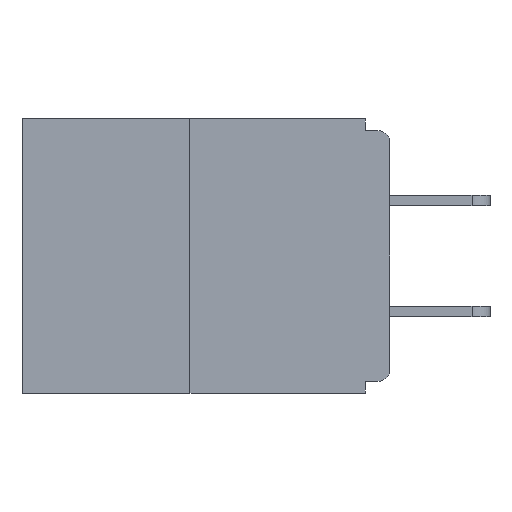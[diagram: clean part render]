
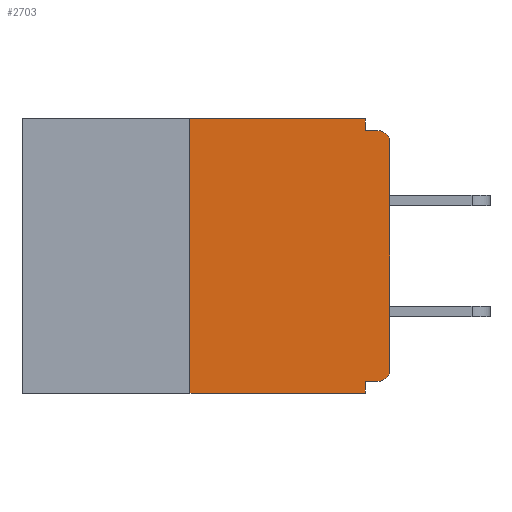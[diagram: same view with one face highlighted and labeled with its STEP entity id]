
A CAD part, left-side view. The second image highlights one B-rep face of the part: STEP entity #2703.
In plain terms, the highlighted planar face has unit normal (-1, 0, 0).
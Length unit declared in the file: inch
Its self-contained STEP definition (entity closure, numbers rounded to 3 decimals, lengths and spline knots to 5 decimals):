
#667 = VECTOR ( 'NONE', #21485, 39.37008 ) ;
#856 = CARTESIAN_POINT ( 'NONE',  ( 0., 0., -0.03 ) ) ;
#1133 = LINE ( 'NONE', #15696, #19356 ) ;
#1563 = CARTESIAN_POINT ( 'NONE',  ( 0., 0.46, 0. ) ) ;
#1723 = AXIS2_PLACEMENT_3D ( 'NONE', #5136, #13846, #15672 ) ;
#2332 = ORIENTED_EDGE ( 'NONE', *, *, #13672, .F. ) ;
#2703 = ADVANCED_FACE ( 'NONE', ( #4633 ), #13112, .F. ) ;
#2776 = LINE ( 'NONE', #4395, #22119 ) ;
#2798 = ORIENTED_EDGE ( 'NONE', *, *, #21049, .F. ) ;
#3098 = VERTEX_POINT ( 'NONE', #856 ) ;
#3648 = DIRECTION ( 'NONE',  ( 0., -1., 0. ) ) ;
#4098 = ORIENTED_EDGE ( 'NONE', *, *, #14912, .F. ) ;
#4188 = VECTOR ( 'NONE', #5619, 39.37008 ) ;
#4358 = EDGE_LOOP ( 'NONE', ( #10697, #2332, #5456, #20576, #17318, #9300, #11180, #11826, #2798, #4098 ) ) ;
#4395 = CARTESIAN_POINT ( 'NONE',  ( 0., 0., 0. ) ) ;
#4628 = DIRECTION ( 'NONE',  ( 0., 0., -1. ) ) ;
#4633 = FACE_OUTER_BOUND ( 'NONE', #4358, .T. ) ;
#4859 = EDGE_CURVE ( 'NONE', #14186, #15803, #20510, .T. ) ;
#5136 = CARTESIAN_POINT ( 'NONE',  ( 0., 0.015, -0.313 ) ) ;
#5456 = ORIENTED_EDGE ( 'NONE', *, *, #11214, .T. ) ;
#5619 = DIRECTION ( 'NONE',  ( 0., 0., -1. ) ) ;
#6028 = CIRCLE ( 'NONE', #17965, 0.015 ) ;
#6370 = DIRECTION ( 'NONE',  ( 1., 0., 0. ) ) ;
#7706 = DIRECTION ( 'NONE',  ( 0., 0., 1. ) ) ;
#7786 = CARTESIAN_POINT ( 'NONE',  ( 0., 0.031, -0.015 ) ) ;
#7933 = VERTEX_POINT ( 'NONE', #12059 ) ;
#8176 = CARTESIAN_POINT ( 'NONE',  ( 0., 0.46, 0. ) ) ;
#8432 = VERTEX_POINT ( 'NONE', #13363 ) ;
#8633 = CARTESIAN_POINT ( 'NONE',  ( 0., 0.031, -0.328 ) ) ;
#9161 = LINE ( 'NONE', #14017, #18125 ) ;
#9219 = VERTEX_POINT ( 'NONE', #19169 ) ;
#9300 = ORIENTED_EDGE ( 'NONE', *, *, #4859, .T. ) ;
#9539 = LINE ( 'NONE', #1563, #13895 ) ;
#10603 = EDGE_CURVE ( 'NONE', #3098, #8432, #6028, .T. ) ;
#10697 = ORIENTED_EDGE ( 'NONE', *, *, #11907, .F. ) ;
#10717 = EDGE_CURVE ( 'NONE', #15803, #3098, #2776, .T. ) ;
#11003 = VERTEX_POINT ( 'NONE', #13660 ) ;
#11180 = ORIENTED_EDGE ( 'NONE', *, *, #10717, .T. ) ;
#11214 = EDGE_CURVE ( 'NONE', #7933, #11003, #1133, .T. ) ;
#11826 = ORIENTED_EDGE ( 'NONE', *, *, #10603, .T. ) ;
#11907 = EDGE_CURVE ( 'NONE', #9219, #16739, #9539, .T. ) ;
#12013 = CARTESIAN_POINT ( 'NONE',  ( 0., 0.031, 0. ) ) ;
#12059 = CARTESIAN_POINT ( 'NONE',  ( 0., 0.25, -0.343 ) ) ;
#12322 = VERTEX_POINT ( 'NONE', #7786 ) ;
#12551 = CARTESIAN_POINT ( 'NONE',  ( 0., 0.031, -0.343 ) ) ;
#13112 = PLANE ( 'NONE',  #17699 ) ;
#13363 = CARTESIAN_POINT ( 'NONE',  ( 0., 0.015, -0.015 ) ) ;
#13660 = CARTESIAN_POINT ( 'NONE',  ( 0., 0.031, -0.343 ) ) ;
#13672 = EDGE_CURVE ( 'NONE', #7933, #9219, #18122, .T. ) ;
#13846 = DIRECTION ( 'NONE',  ( -1., 0., 0. ) ) ;
#13895 = VECTOR ( 'NONE', #17110, 39.37008 ) ;
#14017 = CARTESIAN_POINT ( 'NONE',  ( 0., 0., -0.015 ) ) ;
#14186 = VERTEX_POINT ( 'NONE', #18521 ) ;
#14224 = VECTOR ( 'NONE', #21206, 39.37008 ) ;
#14851 = VERTEX_POINT ( 'NONE', #8633 ) ;
#14912 = EDGE_CURVE ( 'NONE', #16739, #12322, #18078, .T. ) ;
#15378 = LINE ( 'NONE', #12551, #667 ) ;
#15484 = EDGE_CURVE ( 'NONE', #14851, #11003, #15378, .T. ) ;
#15672 = DIRECTION ( 'NONE',  ( 0., 0., -1. ) ) ;
#15696 = CARTESIAN_POINT ( 'NONE',  ( 0., 0.46, -0.343 ) ) ;
#15803 = VERTEX_POINT ( 'NONE', #19522 ) ;
#16241 = DIRECTION ( 'NONE',  ( -1., 0., 0. ) ) ;
#16739 = VERTEX_POINT ( 'NONE', #12013 ) ;
#17110 = DIRECTION ( 'NONE',  ( 0., -1., 0. ) ) ;
#17318 = ORIENTED_EDGE ( 'NONE', *, *, #17610, .F. ) ;
#17483 = DIRECTION ( 'NONE',  ( 0., 0., 1. ) ) ;
#17581 = VECTOR ( 'NONE', #17483, 39.37008 ) ;
#17610 = EDGE_CURVE ( 'NONE', #14186, #14851, #22128, .T. ) ;
#17699 = AXIS2_PLACEMENT_3D ( 'NONE', #8176, #6370, #4628 ) ;
#17965 = AXIS2_PLACEMENT_3D ( 'NONE', #18267, #16241, #18348 ) ;
#18078 = LINE ( 'NONE', #19797, #4188 ) ;
#18122 = LINE ( 'NONE', #20872, #17581 ) ;
#18125 = VECTOR ( 'NONE', #19679, 39.37008 ) ;
#18267 = CARTESIAN_POINT ( 'NONE',  ( 0., 0.015, -0.03 ) ) ;
#18348 = DIRECTION ( 'NONE',  ( 0., 0., -1. ) ) ;
#18521 = CARTESIAN_POINT ( 'NONE',  ( 0., 0.015, -0.328 ) ) ;
#19169 = CARTESIAN_POINT ( 'NONE',  ( 0., 0.25, 0. ) ) ;
#19356 = VECTOR ( 'NONE', #3648, 39.37008 ) ;
#19522 = CARTESIAN_POINT ( 'NONE',  ( 0., 0., -0.313 ) ) ;
#19679 = DIRECTION ( 'NONE',  ( 0., -1., 0. ) ) ;
#19797 = CARTESIAN_POINT ( 'NONE',  ( 0., 0.031, 0. ) ) ;
#20510 = CIRCLE ( 'NONE', #1723, 0.015 ) ;
#20576 = ORIENTED_EDGE ( 'NONE', *, *, #15484, .F. ) ;
#20606 = CARTESIAN_POINT ( 'NONE',  ( 0., 0., -0.328 ) ) ;
#20872 = CARTESIAN_POINT ( 'NONE',  ( 0., 0.25, 0. ) ) ;
#21049 = EDGE_CURVE ( 'NONE', #12322, #8432, #9161, .T. ) ;
#21206 = DIRECTION ( 'NONE',  ( 0., 1., 0. ) ) ;
#21485 = DIRECTION ( 'NONE',  ( 0., 0., -1. ) ) ;
#22119 = VECTOR ( 'NONE', #7706, 39.37008 ) ;
#22128 = LINE ( 'NONE', #20606, #14224 ) ;
